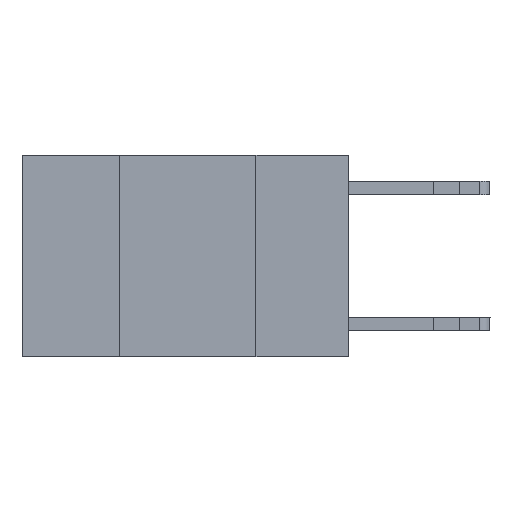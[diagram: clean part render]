
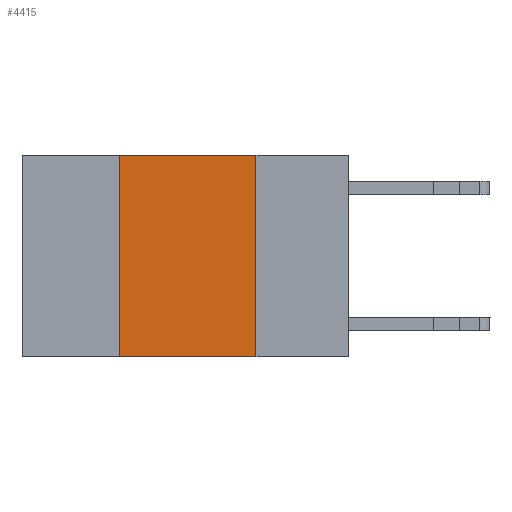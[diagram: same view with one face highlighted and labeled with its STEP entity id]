
A CAD part, left-side view. The second image highlights one B-rep face of the part: STEP entity #4415.
In plain terms, the highlighted planar face has unit normal (-1, 0, 0).
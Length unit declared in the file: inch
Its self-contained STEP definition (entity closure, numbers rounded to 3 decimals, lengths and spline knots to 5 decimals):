
#35 = LINE ( 'NONE', #5863, #12752 ) ;
#199 = VERTEX_POINT ( 'NONE', #10461 ) ;
#207 = EDGE_LOOP ( 'NONE', ( #5655, #8723, #11330, #7125 ) ) ;
#540 = FACE_OUTER_BOUND ( 'NONE', #207, .T. ) ;
#711 = LINE ( 'NONE', #10070, #8688 ) ;
#1054 = EDGE_CURVE ( 'NONE', #7085, #199, #7337, .T. ) ;
#1731 = AXIS2_PLACEMENT_3D ( 'NONE', #11783, #8960, #2595 ) ;
#1856 = CARTESIAN_POINT ( 'NONE',  ( 0., 0.42, 0. ) ) ;
#2595 = DIRECTION ( 'NONE',  ( 0., 0., -1. ) ) ;
#3164 = CARTESIAN_POINT ( 'NONE',  ( 0., 0.6, 0. ) ) ;
#3364 = EDGE_CURVE ( 'NONE', #7570, #7085, #711, .T. ) ;
#4415 = ADVANCED_FACE ( 'NONE', ( #540 ), #7954, .F. ) ;
#4443 = CARTESIAN_POINT ( 'NONE',  ( 0., 0.42, -0.37 ) ) ;
#5097 = CARTESIAN_POINT ( 'NONE',  ( 0., 0.17, -0.37 ) ) ;
#5325 = VECTOR ( 'NONE', #8810, 39.37008 ) ;
#5650 = CARTESIAN_POINT ( 'NONE',  ( 0., 0.17, 0. ) ) ;
#5655 = ORIENTED_EDGE ( 'NONE', *, *, #10085, .F. ) ;
#5863 = CARTESIAN_POINT ( 'NONE',  ( 0., 0.6, -0.37 ) ) ;
#7034 = DIRECTION ( 'NONE',  ( 0., -1., 0. ) ) ;
#7085 = VERTEX_POINT ( 'NONE', #1856 ) ;
#7125 = ORIENTED_EDGE ( 'NONE', *, *, #12178, .T. ) ;
#7337 = LINE ( 'NONE', #3164, #12437 ) ;
#7570 = VERTEX_POINT ( 'NONE', #4443 ) ;
#7954 = PLANE ( 'NONE',  #1731 ) ;
#8688 = VECTOR ( 'NONE', #11027, 39.37008 ) ;
#8723 = ORIENTED_EDGE ( 'NONE', *, *, #1054, .F. ) ;
#8810 = DIRECTION ( 'NONE',  ( 0., 0., -1. ) ) ;
#8833 = LINE ( 'NONE', #5650, #5325 ) ;
#8889 = VERTEX_POINT ( 'NONE', #5097 ) ;
#8960 = DIRECTION ( 'NONE',  ( 1., 0., 0. ) ) ;
#10070 = CARTESIAN_POINT ( 'NONE',  ( 0., 0.42, 0. ) ) ;
#10085 = EDGE_CURVE ( 'NONE', #199, #8889, #8833, .T. ) ;
#10461 = CARTESIAN_POINT ( 'NONE',  ( 0., 0.17, 0. ) ) ;
#10517 = DIRECTION ( 'NONE',  ( 0., -1., 0. ) ) ;
#11027 = DIRECTION ( 'NONE',  ( 0., 0., 1. ) ) ;
#11330 = ORIENTED_EDGE ( 'NONE', *, *, #3364, .F. ) ;
#11783 = CARTESIAN_POINT ( 'NONE',  ( 0., 0.6, 0. ) ) ;
#12178 = EDGE_CURVE ( 'NONE', #7570, #8889, #35, .T. ) ;
#12437 = VECTOR ( 'NONE', #10517, 39.37008 ) ;
#12752 = VECTOR ( 'NONE', #7034, 39.37008 ) ;
